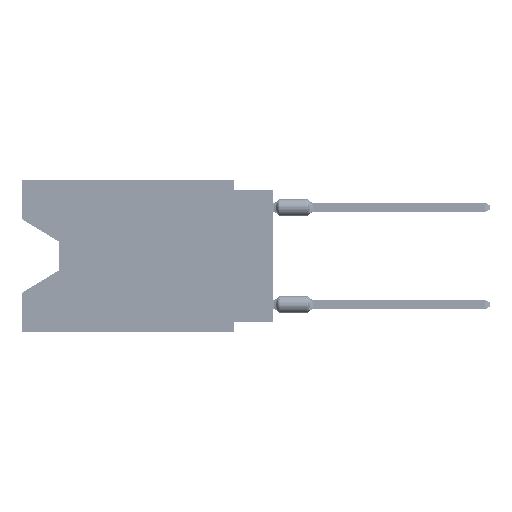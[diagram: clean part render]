
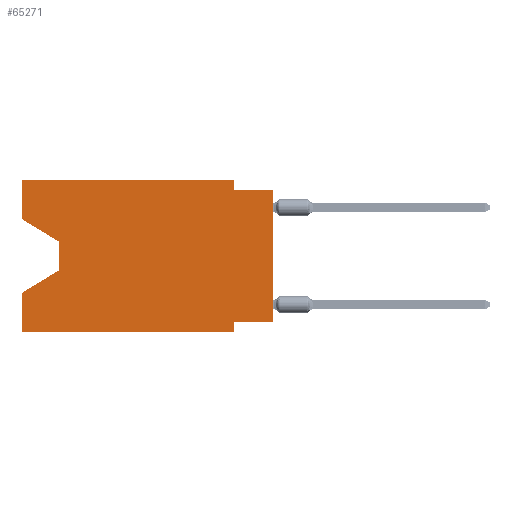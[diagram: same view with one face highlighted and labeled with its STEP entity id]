
A CAD part, left-side view. The second image highlights one B-rep face of the part: STEP entity #65271.
In plain terms, the highlighted planar face has unit normal (-1, 0, 0).
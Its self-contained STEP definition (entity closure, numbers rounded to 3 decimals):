
#1493 = DIRECTION ( 'NONE',  ( 0., 0., 1. ) ) ;
#1964 = CARTESIAN_POINT ( 'NONE',  ( 0., 0., -0.635 ) ) ;
#2881 = DIRECTION ( 'NONE',  ( 0., 0., -1. ) ) ;
#3252 = LINE ( 'NONE', #22814, #8458 ) ;
#6228 = ORIENTED_EDGE ( 'NONE', *, *, #11685, .T. ) ;
#6879 = CARTESIAN_POINT ( 'NONE',  ( 0., 2.54, -9.906 ) ) ;
#7057 = LINE ( 'NONE', #25757, #33657 ) ;
#8361 = ORIENTED_EDGE ( 'NONE', *, *, #16237, .F. ) ;
#8458 = VECTOR ( 'NONE', #36705, 1000. ) ;
#8805 = VECTOR ( 'NONE', #74735, 1000. ) ;
#9338 = VECTOR ( 'NONE', #44408, 1000. ) ;
#9406 = PLANE ( 'NONE',  #23650 ) ;
#9834 = DIRECTION ( 'NONE',  ( 0., -1., 0. ) ) ;
#10261 = LINE ( 'NONE', #71051, #84865 ) ;
#10524 = ORIENTED_EDGE ( 'NONE', *, *, #85353, .T. ) ;
#10534 = LINE ( 'NONE', #42680, #9338 ) ;
#11021 = VERTEX_POINT ( 'NONE', #6879 ) ;
#11606 = ORIENTED_EDGE ( 'NONE', *, *, #17325, .F. ) ;
#11685 = EDGE_CURVE ( 'NONE', #26020, #52208, #3252, .T. ) ;
#11901 = VERTEX_POINT ( 'NONE', #26236 ) ;
#12260 = CARTESIAN_POINT ( 'NONE',  ( 0., 2.54, 0. ) ) ;
#13539 = LINE ( 'NONE', #34358, #8805 ) ;
#14831 = EDGE_LOOP ( 'NONE', ( #35835, #48735, #6228, #35066, #10524, #63007, #18348, #29784, #8361, #21214, #35594, #11606 ) ) ;
#16237 = EDGE_CURVE ( 'NONE', #54485, #77937, #67085, .T. ) ;
#17325 = EDGE_CURVE ( 'NONE', #70702, #11901, #7057, .T. ) ;
#18348 = ORIENTED_EDGE ( 'NONE', *, *, #29179, .F. ) ;
#20717 = CARTESIAN_POINT ( 'NONE',  ( 0., 0., -9.271 ) ) ;
#20948 = CARTESIAN_POINT ( 'NONE',  ( 0., 2.54, -0.635 ) ) ;
#21214 = ORIENTED_EDGE ( 'NONE', *, *, #35509, .F. ) ;
#22164 = CARTESIAN_POINT ( 'NONE',  ( 0., 16.383, -7.36 ) ) ;
#22814 = CARTESIAN_POINT ( 'NONE',  ( 0., 13.97, -5.893 ) ) ;
#23650 = AXIS2_PLACEMENT_3D ( 'NONE', #35903, #62389, #2881 ) ;
#24021 = LINE ( 'NONE', #12260, #56232 ) ;
#25757 = CARTESIAN_POINT ( 'NONE',  ( 0., 16.383, 0. ) ) ;
#26020 = VERTEX_POINT ( 'NONE', #64861 ) ;
#26236 = CARTESIAN_POINT ( 'NONE',  ( 0., 16.383, 0. ) ) ;
#29179 = EDGE_CURVE ( 'NONE', #74190, #58969, #58267, .T. ) ;
#29388 = VECTOR ( 'NONE', #50901, 1000. ) ;
#29784 = ORIENTED_EDGE ( 'NONE', *, *, #59647, .T. ) ;
#30666 = LINE ( 'NONE', #62798, #82004 ) ;
#30712 = EDGE_CURVE ( 'NONE', #58969, #11021, #13539, .T. ) ;
#31896 = VECTOR ( 'NONE', #40168, 1000. ) ;
#32489 = CARTESIAN_POINT ( 'NONE',  ( 0., 13.97, -4.013 ) ) ;
#33219 = CARTESIAN_POINT ( 'NONE',  ( 0., 0., -0.635 ) ) ;
#33657 = VECTOR ( 'NONE', #45748, 1000. ) ;
#34358 = CARTESIAN_POINT ( 'NONE',  ( 0., 2.54, -9.906 ) ) ;
#34522 = LINE ( 'NONE', #61015, #35459 ) ;
#34832 = DIRECTION ( 'NONE',  ( 0., -0.855, -0.519 ) ) ;
#35066 = ORIENTED_EDGE ( 'NONE', *, *, #73566, .F. ) ;
#35258 = LINE ( 'NONE', #82578, #63547 ) ;
#35459 = VECTOR ( 'NONE', #1493, 1000. ) ;
#35509 = EDGE_CURVE ( 'NONE', #65809, #54485, #24021, .T. ) ;
#35594 = ORIENTED_EDGE ( 'NONE', *, *, #37420, .F. ) ;
#35835 = ORIENTED_EDGE ( 'NONE', *, *, #38679, .T. ) ;
#35903 = CARTESIAN_POINT ( 'NONE',  ( 0., 16.383, 0. ) ) ;
#36705 = DIRECTION ( 'NONE',  ( 0., 0.855, -0.519 ) ) ;
#37420 = EDGE_CURVE ( 'NONE', #11901, #65809, #10534, .T. ) ;
#38679 = EDGE_CURVE ( 'NONE', #70702, #64912, #35258, .T. ) ;
#38758 = DIRECTION ( 'NONE',  ( 0., 0., -1. ) ) ;
#40168 = DIRECTION ( 'NONE',  ( 0., -1., 0. ) ) ;
#42680 = CARTESIAN_POINT ( 'NONE',  ( 0., 16.383, 0. ) ) ;
#43524 = CARTESIAN_POINT ( 'NONE',  ( 0., 2.54, -9.271 ) ) ;
#44164 = CARTESIAN_POINT ( 'NONE',  ( 0., 16.383, -9.906 ) ) ;
#44408 = DIRECTION ( 'NONE',  ( 0., -1., 0. ) ) ;
#45748 = DIRECTION ( 'NONE',  ( 0., 0., 1. ) ) ;
#48735 = ORIENTED_EDGE ( 'NONE', *, *, #84100, .T. ) ;
#50018 = DIRECTION ( 'NONE',  ( 0., 0., 1. ) ) ;
#50874 = CARTESIAN_POINT ( 'NONE',  ( 0., 16.383, 0. ) ) ;
#50901 = DIRECTION ( 'NONE',  ( 0., 1., 0. ) ) ;
#52208 = VERTEX_POINT ( 'NONE', #22164 ) ;
#54485 = VERTEX_POINT ( 'NONE', #20948 ) ;
#56232 = VECTOR ( 'NONE', #38758, 1000. ) ;
#57073 = CARTESIAN_POINT ( 'NONE',  ( 0., 2.54, 0. ) ) ;
#58267 = LINE ( 'NONE', #58693, #29388 ) ;
#58693 = CARTESIAN_POINT ( 'NONE',  ( 0., 0., -9.271 ) ) ;
#58969 = VERTEX_POINT ( 'NONE', #43524 ) ;
#59647 = EDGE_CURVE ( 'NONE', #74190, #77937, #34522, .T. ) ;
#61015 = CARTESIAN_POINT ( 'NONE',  ( 0., 0., 0. ) ) ;
#62127 = VECTOR ( 'NONE', #50018, 1000. ) ;
#62389 = DIRECTION ( 'NONE',  ( 1., 0., 0. ) ) ;
#62798 = CARTESIAN_POINT ( 'NONE',  ( 0., 13.97, -4.013 ) ) ;
#63007 = ORIENTED_EDGE ( 'NONE', *, *, #30712, .F. ) ;
#63038 = LINE ( 'NONE', #50874, #62127 ) ;
#63547 = VECTOR ( 'NONE', #34832, 1000. ) ;
#64861 = CARTESIAN_POINT ( 'NONE',  ( 0., 13.97, -5.893 ) ) ;
#64912 = VERTEX_POINT ( 'NONE', #32489 ) ;
#65271 = ADVANCED_FACE ( 'NONE', ( #68906 ), #9406, .F. ) ;
#65809 = VERTEX_POINT ( 'NONE', #57073 ) ;
#67085 = LINE ( 'NONE', #33219, #31896 ) ;
#68906 = FACE_OUTER_BOUND ( 'NONE', #14831, .T. ) ;
#69543 = VERTEX_POINT ( 'NONE', #44164 ) ;
#70702 = VERTEX_POINT ( 'NONE', #78703 ) ;
#71051 = CARTESIAN_POINT ( 'NONE',  ( 0., 16.383, -9.906 ) ) ;
#73566 = EDGE_CURVE ( 'NONE', #69543, #52208, #63038, .T. ) ;
#74190 = VERTEX_POINT ( 'NONE', #20717 ) ;
#74735 = DIRECTION ( 'NONE',  ( 0., 0., -1. ) ) ;
#77937 = VERTEX_POINT ( 'NONE', #1964 ) ;
#78703 = CARTESIAN_POINT ( 'NONE',  ( 0., 16.383, -2.546 ) ) ;
#82004 = VECTOR ( 'NONE', #83631, 1000. ) ;
#82578 = CARTESIAN_POINT ( 'NONE',  ( 0., 16.383, -2.546 ) ) ;
#83631 = DIRECTION ( 'NONE',  ( 0., 0., -1. ) ) ;
#84100 = EDGE_CURVE ( 'NONE', #64912, #26020, #30666, .T. ) ;
#84865 = VECTOR ( 'NONE', #9834, 1000. ) ;
#85353 = EDGE_CURVE ( 'NONE', #69543, #11021, #10261, .T. ) ;
